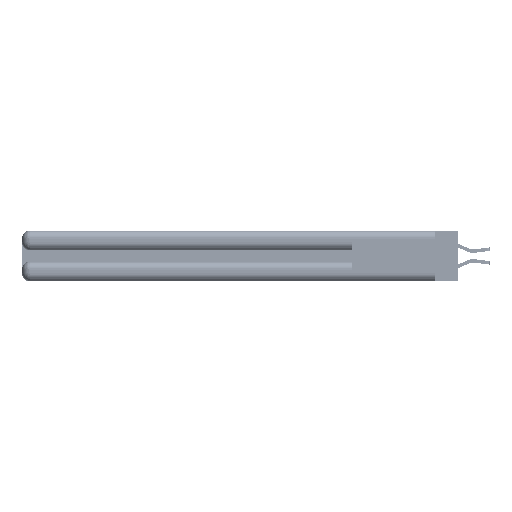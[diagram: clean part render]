
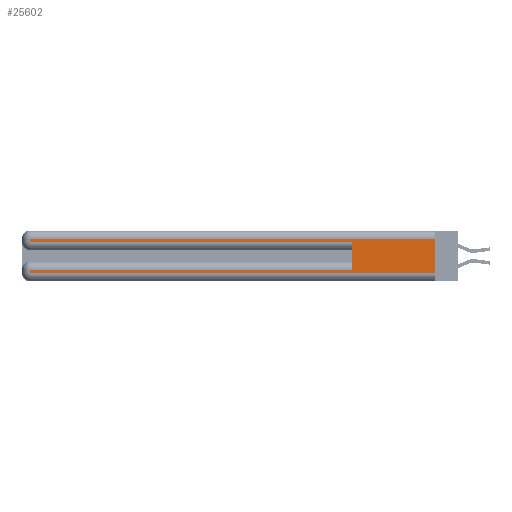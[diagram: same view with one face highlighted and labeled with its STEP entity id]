
A CAD part, left-side view. The second image highlights one B-rep face of the part: STEP entity #25602.
In plain terms, the highlighted planar face has unit normal (-1, 0, 0).
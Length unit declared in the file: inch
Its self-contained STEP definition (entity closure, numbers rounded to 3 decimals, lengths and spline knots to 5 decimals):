
#561 = DIRECTION ( 'NONE',  ( 0., 0., -1. ) ) ;
#914 = CARTESIAN_POINT ( 'NONE',  ( 0., 0., 0.37 ) ) ;
#1013 = VECTOR ( 'NONE', #35267, 39.37008 ) ;
#1532 = ORIENTED_EDGE ( 'NONE', *, *, #6239, .T. ) ;
#2603 = LINE ( 'NONE', #28728, #30900 ) ;
#2721 = CARTESIAN_POINT ( 'NONE',  ( 0., 0., 0.06 ) ) ;
#2907 = CARTESIAN_POINT ( 'NONE',  ( 0., 2.94, 0.31 ) ) ;
#3282 = VERTEX_POINT ( 'NONE', #2907 ) ;
#3640 = LINE ( 'NONE', #3843, #25312 ) ;
#3702 = CARTESIAN_POINT ( 'NONE',  ( 0., 2.94, 0.285 ) ) ;
#3793 = LINE ( 'NONE', #16382, #9845 ) ;
#3843 = CARTESIAN_POINT ( 'NONE',  ( 0., 0., 0.37 ) ) ;
#4410 = VERTEX_POINT ( 'NONE', #39414 ) ;
#4531 = EDGE_CURVE ( 'NONE', #3282, #24312, #3793, .T. ) ;
#5130 = AXIS2_PLACEMENT_3D ( 'NONE', #914, #36924, #7725 ) ;
#5309 = DIRECTION ( 'NONE',  ( 0., 0., 1. ) ) ;
#6239 = EDGE_CURVE ( 'NONE', #12814, #3282, #2603, .T. ) ;
#7725 = DIRECTION ( 'NONE',  ( 0., 0., -1. ) ) ;
#9845 = VECTOR ( 'NONE', #561, 39.37008 ) ;
#10099 = LINE ( 'NONE', #26915, #41452 ) ;
#12294 = VERTEX_POINT ( 'NONE', #2721 ) ;
#12814 = VERTEX_POINT ( 'NONE', #40427 ) ;
#13902 = VECTOR ( 'NONE', #5309, 39.37008 ) ;
#14331 = PLANE ( 'NONE',  #5130 ) ;
#14496 = EDGE_CURVE ( 'NONE', #12814, #12294, #3640, .T. ) ;
#15727 = LINE ( 'NONE', #35610, #21273 ) ;
#16382 = CARTESIAN_POINT ( 'NONE',  ( 0., 2.94, 0.37 ) ) ;
#18618 = ORIENTED_EDGE ( 'NONE', *, *, #4531, .T. ) ;
#18729 = CARTESIAN_POINT ( 'NONE',  ( 0., 0., 0.06 ) ) ;
#19075 = VECTOR ( 'NONE', #29431, 39.37008 ) ;
#19537 = DIRECTION ( 'NONE',  ( 0., 0., -1. ) ) ;
#20772 = ORIENTED_EDGE ( 'NONE', *, *, #38715, .T. ) ;
#21166 = ORIENTED_EDGE ( 'NONE', *, *, #14496, .F. ) ;
#21273 = VECTOR ( 'NONE', #39133, 39.37008 ) ;
#24312 = VERTEX_POINT ( 'NONE', #3702 ) ;
#24779 = CARTESIAN_POINT ( 'NONE',  ( 0., 0.6, 0.145 ) ) ;
#24812 = ORIENTED_EDGE ( 'NONE', *, *, #33825, .T. ) ;
#25063 = EDGE_LOOP ( 'NONE', ( #21166, #1532, #18618, #24812, #25516, #25224, #20772, #38339 ) ) ;
#25224 = ORIENTED_EDGE ( 'NONE', *, *, #37843, .T. ) ;
#25312 = VECTOR ( 'NONE', #19537, 39.37008 ) ;
#25516 = ORIENTED_EDGE ( 'NONE', *, *, #35513, .F. ) ;
#25602 = ADVANCED_FACE ( 'NONE', ( #25785 ), #14331, .F. ) ;
#25780 = LINE ( 'NONE', #18729, #1013 ) ;
#25785 = FACE_OUTER_BOUND ( 'NONE', #25063, .T. ) ;
#26911 = CARTESIAN_POINT ( 'NONE',  ( 0., 0.6, 0.285 ) ) ;
#26915 = CARTESIAN_POINT ( 'NONE',  ( 0., 2.94, 0.37 ) ) ;
#28728 = CARTESIAN_POINT ( 'NONE',  ( 0., 0., 0.31 ) ) ;
#29388 = CARTESIAN_POINT ( 'NONE',  ( 0., 2.94, 0.06 ) ) ;
#29431 = DIRECTION ( 'NONE',  ( 0., -1., 0. ) ) ;
#30900 = VECTOR ( 'NONE', #35676, 39.37008 ) ;
#30966 = CARTESIAN_POINT ( 'NONE',  ( 0., 2.94, 0.085 ) ) ;
#32802 = VERTEX_POINT ( 'NONE', #26911 ) ;
#33663 = LINE ( 'NONE', #24779, #13902 ) ;
#33696 = DIRECTION ( 'NONE',  ( 0., 0., -1. ) ) ;
#33825 = EDGE_CURVE ( 'NONE', #24312, #32802, #37766, .T. ) ;
#35267 = DIRECTION ( 'NONE',  ( 0., -1., 0. ) ) ;
#35513 = EDGE_CURVE ( 'NONE', #4410, #32802, #33663, .T. ) ;
#35610 = CARTESIAN_POINT ( 'NONE',  ( 0., 0., 0.085 ) ) ;
#35676 = DIRECTION ( 'NONE',  ( 0., 1., 0. ) ) ;
#36924 = DIRECTION ( 'NONE',  ( 1., 0., 0. ) ) ;
#37766 = LINE ( 'NONE', #38219, #19075 ) ;
#37843 = EDGE_CURVE ( 'NONE', #4410, #40181, #15727, .T. ) ;
#38219 = CARTESIAN_POINT ( 'NONE',  ( 0., 0., 0.285 ) ) ;
#38339 = ORIENTED_EDGE ( 'NONE', *, *, #38405, .T. ) ;
#38405 = EDGE_CURVE ( 'NONE', #40425, #12294, #25780, .T. ) ;
#38715 = EDGE_CURVE ( 'NONE', #40181, #40425, #10099, .T. ) ;
#39133 = DIRECTION ( 'NONE',  ( 0., 1., 0. ) ) ;
#39414 = CARTESIAN_POINT ( 'NONE',  ( 0., 0.6, 0.085 ) ) ;
#40181 = VERTEX_POINT ( 'NONE', #30966 ) ;
#40425 = VERTEX_POINT ( 'NONE', #29388 ) ;
#40427 = CARTESIAN_POINT ( 'NONE',  ( 0., 0., 0.31 ) ) ;
#41452 = VECTOR ( 'NONE', #33696, 39.37008 ) ;
